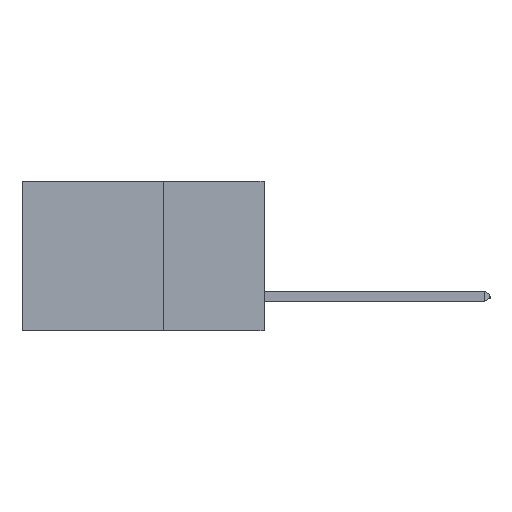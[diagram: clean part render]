
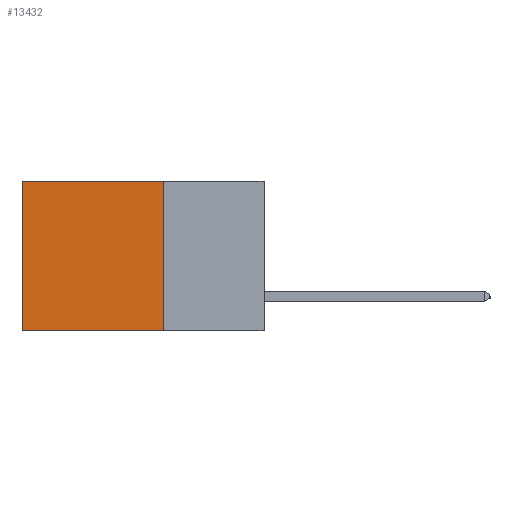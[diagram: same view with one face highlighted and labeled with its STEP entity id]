
A CAD part, left-side view. The second image highlights one B-rep face of the part: STEP entity #13432.
In plain terms, the highlighted planar face has unit normal (-1, 0, 0).
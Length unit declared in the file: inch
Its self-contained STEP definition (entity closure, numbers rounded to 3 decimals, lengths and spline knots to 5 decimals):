
#1320 = ORIENTED_EDGE ( 'NONE', *, *, #4997, .T. ) ;
#1570 = CARTESIAN_POINT ( 'NONE',  ( 0.298, 0.25, 0. ) ) ;
#2000 = EDGE_CURVE ( 'NONE', #3815, #11343, #13553, .T. ) ;
#2844 = LINE ( 'NONE', #5649, #14993 ) ;
#2924 = ORIENTED_EDGE ( 'NONE', *, *, #6931, .T. ) ;
#3187 = EDGE_LOOP ( 'NONE', ( #2924, #6584, #13992, #1320 ) ) ;
#3815 = VERTEX_POINT ( 'NONE', #9202 ) ;
#4050 = LINE ( 'NONE', #11379, #9942 ) ;
#4358 = PLANE ( 'NONE',  #14926 ) ;
#4997 = EDGE_CURVE ( 'NONE', #5466, #13394, #4050, .T. ) ;
#5466 = VERTEX_POINT ( 'NONE', #1570 ) ;
#5649 = CARTESIAN_POINT ( 'NONE',  ( 0.298, 0.25, 0. ) ) ;
#5731 = CARTESIAN_POINT ( 'NONE',  ( 0.298, 0.6, 0. ) ) ;
#6584 = ORIENTED_EDGE ( 'NONE', *, *, #2000, .F. ) ;
#6707 = CARTESIAN_POINT ( 'NONE',  ( 0.298, 0.25, 0. ) ) ;
#6931 = EDGE_CURVE ( 'NONE', #13394, #11343, #15036, .T. ) ;
#7895 = DIRECTION ( 'NONE',  ( 0., 0., -1. ) ) ;
#9202 = CARTESIAN_POINT ( 'NONE',  ( 0.298, 0.25, -0.37 ) ) ;
#9942 = VECTOR ( 'NONE', #14878, 39.37008 ) ;
#10307 = CARTESIAN_POINT ( 'NONE',  ( 0.298, 0.25, -0.37 ) ) ;
#10392 = DIRECTION ( 'NONE',  ( 0., 0., -1. ) ) ;
#10428 = VECTOR ( 'NONE', #12242, 39.37008 ) ;
#10439 = EDGE_CURVE ( 'NONE', #5466, #3815, #2844, .T. ) ;
#11343 = VERTEX_POINT ( 'NONE', #11985 ) ;
#11379 = CARTESIAN_POINT ( 'NONE',  ( 0.298, 0.25, 0. ) ) ;
#11985 = CARTESIAN_POINT ( 'NONE',  ( 0.298, 0.6, -0.37 ) ) ;
#12230 = FACE_OUTER_BOUND ( 'NONE', #3187, .T. ) ;
#12242 = DIRECTION ( 'NONE',  ( 0., 1., 0. ) ) ;
#12323 = VECTOR ( 'NONE', #13961, 39.37008 ) ;
#13394 = VERTEX_POINT ( 'NONE', #14849 ) ;
#13432 = ADVANCED_FACE ( 'NONE', ( #12230 ), #4358, .F. ) ;
#13553 = LINE ( 'NONE', #10307, #10428 ) ;
#13961 = DIRECTION ( 'NONE',  ( 0., 0., -1. ) ) ;
#13992 = ORIENTED_EDGE ( 'NONE', *, *, #10439, .F. ) ;
#14849 = CARTESIAN_POINT ( 'NONE',  ( 0.298, 0.6, 0. ) ) ;
#14878 = DIRECTION ( 'NONE',  ( 0., 1., 0. ) ) ;
#14926 = AXIS2_PLACEMENT_3D ( 'NONE', #6707, #14945, #7895 ) ;
#14945 = DIRECTION ( 'NONE',  ( 1., 0., 0. ) ) ;
#14993 = VECTOR ( 'NONE', #10392, 39.37008 ) ;
#15036 = LINE ( 'NONE', #5731, #12323 ) ;
